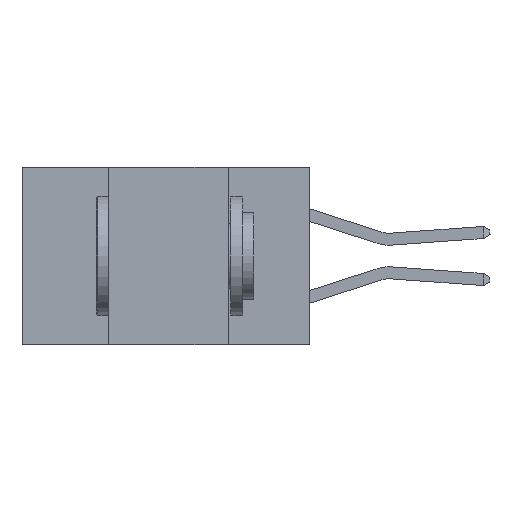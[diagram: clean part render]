
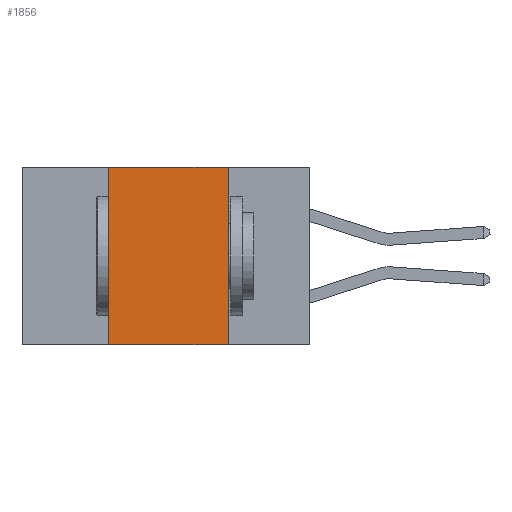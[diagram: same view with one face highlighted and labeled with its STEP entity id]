
A CAD part, left-side view. The second image highlights one B-rep face of the part: STEP entity #1856.
In plain terms, the highlighted planar face has unit normal (-1, 0, 0).
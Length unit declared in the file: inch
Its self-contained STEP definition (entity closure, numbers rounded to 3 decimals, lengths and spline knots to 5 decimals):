
#1418 = EDGE_CURVE ( 'NONE', #5094, #19947, #11490, .T. ) ;
#1829 = DIRECTION ( 'NONE',  ( 0., -1., 0. ) ) ;
#1856 = ADVANCED_FACE ( 'NONE', ( #19175 ), #3189, .F. ) ;
#2269 = VECTOR ( 'NONE', #20434, 39.37008 ) ;
#3119 = DIRECTION ( 'NONE',  ( 0., 0., 1. ) ) ;
#3189 = PLANE ( 'NONE',  #19246 ) ;
#5094 = VERTEX_POINT ( 'NONE', #19310 ) ;
#5232 = ORIENTED_EDGE ( 'NONE', *, *, #7087, .T. ) ;
#5240 = CARTESIAN_POINT ( 'NONE',  ( 0., 0.17, 0. ) ) ;
#5538 = ORIENTED_EDGE ( 'NONE', *, *, #17986, .F. ) ;
#6175 = VECTOR ( 'NONE', #7579, 39.37008 ) ;
#6244 = CARTESIAN_POINT ( 'NONE',  ( 0., 0.42, 0. ) ) ;
#6299 = EDGE_LOOP ( 'NONE', ( #5538, #7107, #8012, #5232 ) ) ;
#6779 = CARTESIAN_POINT ( 'NONE',  ( 0., 0.6, -0.37 ) ) ;
#7087 = EDGE_CURVE ( 'NONE', #5094, #15831, #9860, .T. ) ;
#7107 = ORIENTED_EDGE ( 'NONE', *, *, #13638, .F. ) ;
#7579 = DIRECTION ( 'NONE',  ( 0., 0., -1. ) ) ;
#7673 = CARTESIAN_POINT ( 'NONE',  ( 0., 0.6, 0. ) ) ;
#8012 = ORIENTED_EDGE ( 'NONE', *, *, #1418, .F. ) ;
#8465 = CARTESIAN_POINT ( 'NONE',  ( 0., 0.17, -0.37 ) ) ;
#8564 = DIRECTION ( 'NONE',  ( 1., 0., 0. ) ) ;
#8984 = VECTOR ( 'NONE', #1829, 39.37008 ) ;
#9261 = CARTESIAN_POINT ( 'NONE',  ( 0., 0.17, -0.37 ) ) ;
#9533 = VECTOR ( 'NONE', #3119, 39.37008 ) ;
#9860 = LINE ( 'NONE', #6779, #8984 ) ;
#10402 = VERTEX_POINT ( 'NONE', #5240 ) ;
#10744 = LINE ( 'NONE', #9261, #6175 ) ;
#11490 = LINE ( 'NONE', #14721, #9533 ) ;
#13638 = EDGE_CURVE ( 'NONE', #19947, #10402, #13972, .T. ) ;
#13972 = LINE ( 'NONE', #7673, #2269 ) ;
#14721 = CARTESIAN_POINT ( 'NONE',  ( 0., 0.42, -0.37 ) ) ;
#15831 = VERTEX_POINT ( 'NONE', #8465 ) ;
#16036 = DIRECTION ( 'NONE',  ( 0., 0., -1. ) ) ;
#17603 = CARTESIAN_POINT ( 'NONE',  ( 0., 0.6, 0. ) ) ;
#17986 = EDGE_CURVE ( 'NONE', #10402, #15831, #10744, .T. ) ;
#19175 = FACE_OUTER_BOUND ( 'NONE', #6299, .T. ) ;
#19246 = AXIS2_PLACEMENT_3D ( 'NONE', #17603, #8564, #16036 ) ;
#19310 = CARTESIAN_POINT ( 'NONE',  ( 0., 0.42, -0.37 ) ) ;
#19947 = VERTEX_POINT ( 'NONE', #6244 ) ;
#20434 = DIRECTION ( 'NONE',  ( 0., -1., 0. ) ) ;
